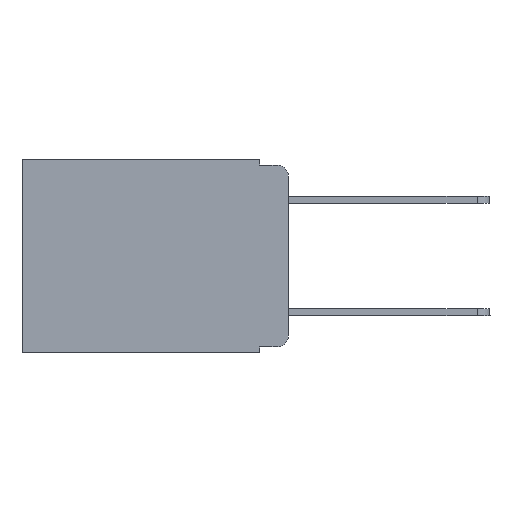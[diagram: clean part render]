
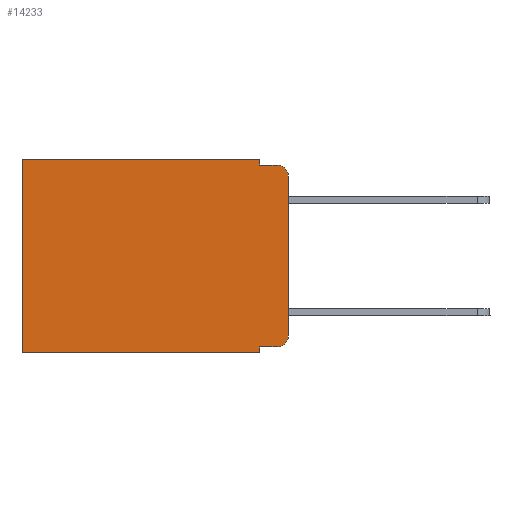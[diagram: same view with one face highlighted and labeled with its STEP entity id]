
A CAD part, left-side view. The second image highlights one B-rep face of the part: STEP entity #14233.
In plain terms, the highlighted planar face has unit normal (-1, 0, 0).
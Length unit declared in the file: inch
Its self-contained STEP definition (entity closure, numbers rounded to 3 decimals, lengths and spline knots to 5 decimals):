
#522 = VERTEX_POINT ( 'NONE', #9203 ) ;
#570 = CARTESIAN_POINT ( 'NONE',  ( 0.298, 0., -0.03 ) ) ;
#700 = LINE ( 'NONE', #1908, #1155 ) ;
#1155 = VECTOR ( 'NONE', #4806, 39.37008 ) ;
#1349 = DIRECTION ( 'NONE',  ( 0., 0., -1. ) ) ;
#1387 = VECTOR ( 'NONE', #7561, 39.37008 ) ;
#1558 = DIRECTION ( 'NONE',  ( 0., 0., -1. ) ) ;
#1908 = CARTESIAN_POINT ( 'NONE',  ( 0.298, 0.051, 0. ) ) ;
#2535 = VERTEX_POINT ( 'NONE', #12228 ) ;
#2573 = LINE ( 'NONE', #10414, #1387 ) ;
#2747 = ORIENTED_EDGE ( 'NONE', *, *, #3417, .F. ) ;
#2875 = AXIS2_PLACEMENT_3D ( 'NONE', #4463, #3153, #13725 ) ;
#3018 = CARTESIAN_POINT ( 'NONE',  ( 0.298, 0.02, -0.01 ) ) ;
#3153 = DIRECTION ( 'NONE',  ( -1., 0., 0. ) ) ;
#3178 = EDGE_CURVE ( 'NONE', #2535, #6746, #4848, .T. ) ;
#3417 = EDGE_CURVE ( 'NONE', #2535, #6584, #9517, .T. ) ;
#3494 = LINE ( 'NONE', #12500, #6997 ) ;
#3532 = DIRECTION ( 'NONE',  ( 0., -1., 0. ) ) ;
#3631 = ORIENTED_EDGE ( 'NONE', *, *, #9990, .T. ) ;
#3803 = CARTESIAN_POINT ( 'NONE',  ( 0.298, 0.051, -0.343 ) ) ;
#3971 = DIRECTION ( 'NONE',  ( -1., 0., 0. ) ) ;
#3986 = DIRECTION ( 'NONE',  ( 0., 0., -1. ) ) ;
#4222 = CARTESIAN_POINT ( 'NONE',  ( 0.298, 0.02, -0.333 ) ) ;
#4286 = VERTEX_POINT ( 'NONE', #3018 ) ;
#4302 = VERTEX_POINT ( 'NONE', #14898 ) ;
#4463 = CARTESIAN_POINT ( 'NONE',  ( 0.298, 0.02, -0.313 ) ) ;
#4795 = VECTOR ( 'NONE', #3986, 39.37008 ) ;
#4806 = DIRECTION ( 'NONE',  ( 0., 0., -1. ) ) ;
#4848 = LINE ( 'NONE', #10143, #16876 ) ;
#5193 = EDGE_CURVE ( 'NONE', #6746, #10502, #15334, .T. ) ;
#5309 = LINE ( 'NONE', #13175, #15041 ) ;
#6111 = EDGE_CURVE ( 'NONE', #16147, #10502, #9042, .T. ) ;
#6220 = EDGE_CURVE ( 'NONE', #15404, #4286, #5309, .T. ) ;
#6584 = VERTEX_POINT ( 'NONE', #3803 ) ;
#6586 = LINE ( 'NONE', #13157, #14388 ) ;
#6746 = VERTEX_POINT ( 'NONE', #4222 ) ;
#6994 = ORIENTED_EDGE ( 'NONE', *, *, #13832, .F. ) ;
#6997 = VECTOR ( 'NONE', #7333, 39.37008 ) ;
#7060 = ORIENTED_EDGE ( 'NONE', *, *, #6220, .F. ) ;
#7238 = VECTOR ( 'NONE', #14876, 39.37008 ) ;
#7333 = DIRECTION ( 'NONE',  ( 0., 1., 0. ) ) ;
#7561 = DIRECTION ( 'NONE',  ( 0., 1., 0. ) ) ;
#8217 = CARTESIAN_POINT ( 'NONE',  ( 0.298, 0.051, 0. ) ) ;
#8276 = ORIENTED_EDGE ( 'NONE', *, *, #3178, .T. ) ;
#9042 = LINE ( 'NONE', #14306, #4795 ) ;
#9203 = CARTESIAN_POINT ( 'NONE',  ( 0.298, 0.051, 0. ) ) ;
#9249 = CARTESIAN_POINT ( 'NONE',  ( 0.298, 0.473, 0. ) ) ;
#9517 = LINE ( 'NONE', #8217, #7238 ) ;
#9530 = CARTESIAN_POINT ( 'NONE',  ( 0.298, 0.02, -0.03 ) ) ;
#9601 = ORIENTED_EDGE ( 'NONE', *, *, #13854, .F. ) ;
#9665 = ORIENTED_EDGE ( 'NONE', *, *, #5193, .T. ) ;
#9838 = ORIENTED_EDGE ( 'NONE', *, *, #12446, .T. ) ;
#9943 = EDGE_CURVE ( 'NONE', #16147, #4286, #16030, .T. ) ;
#9990 = EDGE_CURVE ( 'NONE', #14976, #4302, #6586, .T. ) ;
#10143 = CARTESIAN_POINT ( 'NONE',  ( 0.298, 0.051, -0.333 ) ) ;
#10414 = CARTESIAN_POINT ( 'NONE',  ( 0.298, 0., 0. ) ) ;
#10502 = VERTEX_POINT ( 'NONE', #13963 ) ;
#10579 = DIRECTION ( 'NONE',  ( 0., -1., 0. ) ) ;
#10886 = EDGE_LOOP ( 'NONE', ( #13209, #16192, #7060, #9601, #9838, #3631, #6994, #2747, #8276, #9665 ) ) ;
#12147 = FACE_OUTER_BOUND ( 'NONE', #10886, .T. ) ;
#12174 = AXIS2_PLACEMENT_3D ( 'NONE', #9530, #3971, #14546 ) ;
#12228 = CARTESIAN_POINT ( 'NONE',  ( 0.298, 0.051, -0.333 ) ) ;
#12232 = CARTESIAN_POINT ( 'NONE',  ( 0.298, 0., 0. ) ) ;
#12446 = EDGE_CURVE ( 'NONE', #522, #14976, #2573, .T. ) ;
#12500 = CARTESIAN_POINT ( 'NONE',  ( 0.298, 0., -0.343 ) ) ;
#12509 = AXIS2_PLACEMENT_3D ( 'NONE', #12232, #13613, #1558 ) ;
#13157 = CARTESIAN_POINT ( 'NONE',  ( 0.298, 0.473, 0. ) ) ;
#13175 = CARTESIAN_POINT ( 'NONE',  ( 0.298, 0.051, -0.01 ) ) ;
#13209 = ORIENTED_EDGE ( 'NONE', *, *, #6111, .F. ) ;
#13362 = CARTESIAN_POINT ( 'NONE',  ( 0.298, 0.051, -0.01 ) ) ;
#13449 = PLANE ( 'NONE',  #12509 ) ;
#13613 = DIRECTION ( 'NONE',  ( 1., 0., 0. ) ) ;
#13725 = DIRECTION ( 'NONE',  ( 0., 0., -1. ) ) ;
#13832 = EDGE_CURVE ( 'NONE', #6584, #4302, #3494, .T. ) ;
#13854 = EDGE_CURVE ( 'NONE', #522, #15404, #700, .T. ) ;
#13963 = CARTESIAN_POINT ( 'NONE',  ( 0.298, 0., -0.313 ) ) ;
#14233 = ADVANCED_FACE ( 'NONE', ( #12147 ), #13449, .F. ) ;
#14306 = CARTESIAN_POINT ( 'NONE',  ( 0.298, 0., 0. ) ) ;
#14388 = VECTOR ( 'NONE', #1349, 39.37008 ) ;
#14546 = DIRECTION ( 'NONE',  ( 0., 0., -1. ) ) ;
#14876 = DIRECTION ( 'NONE',  ( 0., 0., -1. ) ) ;
#14898 = CARTESIAN_POINT ( 'NONE',  ( 0.298, 0.473, -0.343 ) ) ;
#14976 = VERTEX_POINT ( 'NONE', #9249 ) ;
#15041 = VECTOR ( 'NONE', #10579, 39.37008 ) ;
#15334 = CIRCLE ( 'NONE', #2875, 0.02 ) ;
#15404 = VERTEX_POINT ( 'NONE', #13362 ) ;
#16030 = CIRCLE ( 'NONE', #12174, 0.02 ) ;
#16147 = VERTEX_POINT ( 'NONE', #570 ) ;
#16192 = ORIENTED_EDGE ( 'NONE', *, *, #9943, .T. ) ;
#16876 = VECTOR ( 'NONE', #3532, 39.37008 ) ;
